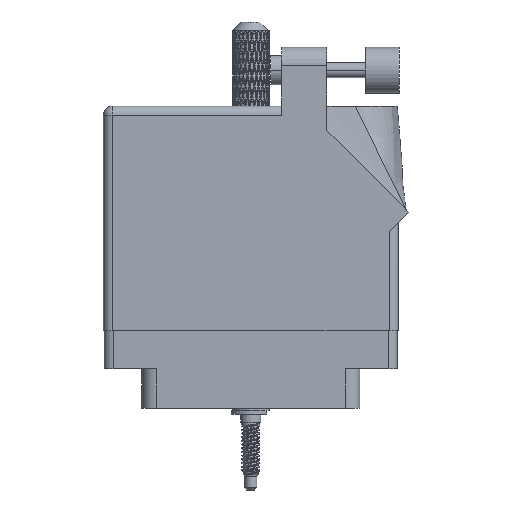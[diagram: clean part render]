
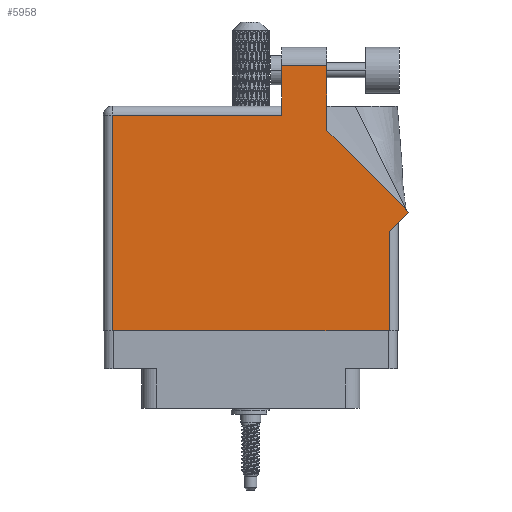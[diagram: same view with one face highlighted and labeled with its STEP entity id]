
A CAD part, front view. The second image highlights one B-rep face of the part: STEP entity #5958.
In plain terms, the highlighted face is planar.
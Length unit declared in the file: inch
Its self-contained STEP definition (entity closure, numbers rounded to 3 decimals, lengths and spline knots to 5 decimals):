
#876 = LINE ( 'NONE', #50414, #32520 ) ;
#1441 = EDGE_CURVE ( 'NONE', #56803, #5247, #55630, .T. ) ;
#3085 = CARTESIAN_POINT ( 'NONE',  ( 1.524, 1.36442, 0. ) ) ;
#3781 = CARTESIAN_POINT ( 'NONE',  ( 1.217, 1.53, 0. ) ) ;
#3835 = VECTOR ( 'NONE', #65738, 39.37008 ) ;
#4266 = EDGE_CURVE ( 'NONE', #36331, #82453, #876, .T. ) ;
#4908 = DIRECTION ( 'NONE',  ( -1., 0., 0. ) ) ;
#5247 = VERTEX_POINT ( 'NONE', #35980 ) ;
#5958 = ADVANCED_FACE ( 'NONE', ( #44921 ), #9968, .F. ) ;
#6352 = VERTEX_POINT ( 'NONE', #79511 ) ;
#8910 = DIRECTION ( 'NONE',  ( 0., 0., -1. ) ) ;
#9554 = ORIENTED_EDGE ( 'NONE', *, *, #27957, .T. ) ;
#9968 = PLANE ( 'NONE',  #20450 ) ;
#12660 = VECTOR ( 'NONE', #90998, 39.37008 ) ;
#17058 = CARTESIAN_POINT ( 'NONE',  ( 0., 1.468, 0. ) ) ;
#17406 = DIRECTION ( 'NONE',  ( 0., 1., 0. ) ) ;
#17553 = EDGE_CURVE ( 'NONE', #5247, #45965, #89255, .T. ) ;
#20450 = AXIS2_PLACEMENT_3D ( 'NONE', #49553, #8910, #81757 ) ;
#21722 = CARTESIAN_POINT ( 'NONE',  ( 1.524, 1.805, 0. ) ) ;
#23773 = VECTOR ( 'NONE', #47419, 39.37008 ) ;
#24278 = EDGE_LOOP ( 'NONE', ( #102173, #9554, #43176, #102733, #104485, #101555, #76440, #27322, #50977 ) ) ;
#24830 = LINE ( 'NONE', #70754, #55173 ) ;
#27322 = ORIENTED_EDGE ( 'NONE', *, *, #42262, .T. ) ;
#27957 = EDGE_CURVE ( 'NONE', #46069, #6352, #104207, .T. ) ;
#28020 = VECTOR ( 'NONE', #44413, 39.37008 ) ;
#32520 = VECTOR ( 'NONE', #57836, 39.37008 ) ;
#34437 = CARTESIAN_POINT ( 'NONE',  ( 1.524, 1.36442, 0. ) ) ;
#35980 = CARTESIAN_POINT ( 'NONE',  ( 1.948, 0., 0. ) ) ;
#36331 = VERTEX_POINT ( 'NONE', #73043 ) ;
#39781 = EDGE_CURVE ( 'NONE', #6352, #76894, #83725, .T. ) ;
#40437 = EDGE_CURVE ( 'NONE', #76894, #40665, #44335, .T. ) ;
#40665 = VERTEX_POINT ( 'NONE', #102722 ) ;
#42262 = EDGE_CURVE ( 'NONE', #45965, #36331, #90900, .T. ) ;
#43176 = ORIENTED_EDGE ( 'NONE', *, *, #39781, .T. ) ;
#44335 = LINE ( 'NONE', #17058, #12660 ) ;
#44413 = DIRECTION ( 'NONE',  ( 0., -1., 0. ) ) ;
#44921 = FACE_OUTER_BOUND ( 'NONE', #24278, .T. ) ;
#45965 = VERTEX_POINT ( 'NONE', #68729 ) ;
#46069 = VERTEX_POINT ( 'NONE', #21722 ) ;
#47147 = DIRECTION ( 'NONE',  ( 0., -1., 0. ) ) ;
#47419 = DIRECTION ( 'NONE',  ( 0.707, 0.707, 0. ) ) ;
#49553 = CARTESIAN_POINT ( 'NONE',  ( 0., 1.53, 0. ) ) ;
#50414 = CARTESIAN_POINT ( 'NONE',  ( 2.08071, 0.80771, 0. ) ) ;
#50977 = ORIENTED_EDGE ( 'NONE', *, *, #4266, .T. ) ;
#55173 = VECTOR ( 'NONE', #47147, 39.37008 ) ;
#55630 = LINE ( 'NONE', #97636, #3835 ) ;
#56384 = EDGE_CURVE ( 'NONE', #40665, #56803, #24830, .T. ) ;
#56803 = VERTEX_POINT ( 'NONE', #73380 ) ;
#57836 = DIRECTION ( 'NONE',  ( -0.707, 0.707, 0. ) ) ;
#61957 = DIRECTION ( 'NONE',  ( 0., 1., 0. ) ) ;
#64603 = VECTOR ( 'NONE', #17406, 39.37008 ) ;
#65738 = DIRECTION ( 'NONE',  ( 1., 0., 0. ) ) ;
#68729 = CARTESIAN_POINT ( 'NONE',  ( 1.948, 0.675, 0. ) ) ;
#70011 = CARTESIAN_POINT ( 'NONE',  ( 1.948, 0.737, 0. ) ) ;
#70754 = CARTESIAN_POINT ( 'NONE',  ( 0.062, 0., 0. ) ) ;
#71512 = VECTOR ( 'NONE', #61957, 39.37008 ) ;
#73043 = CARTESIAN_POINT ( 'NONE',  ( 2.08071, 0.80771, 0. ) ) ;
#73380 = CARTESIAN_POINT ( 'NONE',  ( 0.062, 0., 0. ) ) ;
#75897 = LINE ( 'NONE', #34437, #64603 ) ;
#76440 = ORIENTED_EDGE ( 'NONE', *, *, #17553, .T. ) ;
#76894 = VERTEX_POINT ( 'NONE', #85489 ) ;
#77822 = CARTESIAN_POINT ( 'NONE',  ( 2.01, 0.737, 0. ) ) ;
#79511 = CARTESIAN_POINT ( 'NONE',  ( 1.217, 1.805, 0. ) ) ;
#81757 = DIRECTION ( 'NONE',  ( -1., 0., 0. ) ) ;
#82453 = VERTEX_POINT ( 'NONE', #3085 ) ;
#83725 = LINE ( 'NONE', #3781, #28020 ) ;
#85489 = CARTESIAN_POINT ( 'NONE',  ( 1.217, 1.468, 0. ) ) ;
#85899 = CARTESIAN_POINT ( 'NONE',  ( 1.217, 1.805, 0. ) ) ;
#89255 = LINE ( 'NONE', #70011, #71512 ) ;
#90219 = VECTOR ( 'NONE', #4908, 39.37008 ) ;
#90900 = LINE ( 'NONE', #77822, #23773 ) ;
#90998 = DIRECTION ( 'NONE',  ( -1., 0., 0. ) ) ;
#93292 = EDGE_CURVE ( 'NONE', #82453, #46069, #75897, .T. ) ;
#97636 = CARTESIAN_POINT ( 'NONE',  ( 0., 0., 0. ) ) ;
#101555 = ORIENTED_EDGE ( 'NONE', *, *, #1441, .T. ) ;
#102173 = ORIENTED_EDGE ( 'NONE', *, *, #93292, .T. ) ;
#102722 = CARTESIAN_POINT ( 'NONE',  ( 0.062, 1.468, 0. ) ) ;
#102733 = ORIENTED_EDGE ( 'NONE', *, *, #40437, .T. ) ;
#104207 = LINE ( 'NONE', #85899, #90219 ) ;
#104485 = ORIENTED_EDGE ( 'NONE', *, *, #56384, .T. ) ;
